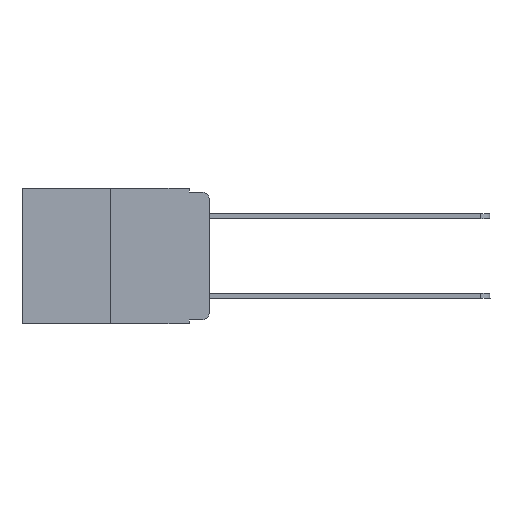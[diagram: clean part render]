
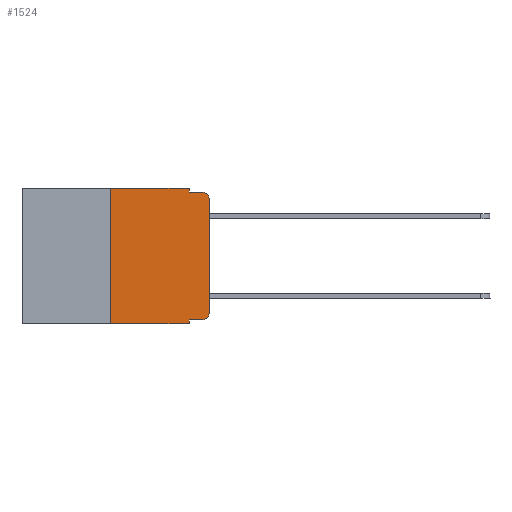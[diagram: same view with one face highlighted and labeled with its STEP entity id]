
A CAD part, left-side view. The second image highlights one B-rep face of the part: STEP entity #1524.
In plain terms, the highlighted planar face has unit normal (-1, 0, 0).
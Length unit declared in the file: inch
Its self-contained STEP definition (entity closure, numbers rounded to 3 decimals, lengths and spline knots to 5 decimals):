
#225 = CARTESIAN_POINT ( 'NONE',  ( 0., 0.473, -0.343 ) ) ;
#423 = VECTOR ( 'NONE', #4324, 39.37008 ) ;
#440 = VERTEX_POINT ( 'NONE', #7628 ) ;
#441 = VERTEX_POINT ( 'NONE', #1644 ) ;
#638 = DIRECTION ( 'NONE',  ( 0., -1., 0. ) ) ;
#814 = AXIS2_PLACEMENT_3D ( 'NONE', #3698, #3149, #5276 ) ;
#901 = EDGE_CURVE ( 'NONE', #3537, #441, #5194, .T. ) ;
#906 = AXIS2_PLACEMENT_3D ( 'NONE', #5093, #6842, #1493 ) ;
#969 = LINE ( 'NONE', #225, #7710 ) ;
#971 = CARTESIAN_POINT ( 'NONE',  ( 0., 0.051, -0.343 ) ) ;
#973 = CARTESIAN_POINT ( 'NONE',  ( 0., 0.051, 0. ) ) ;
#1084 = ORIENTED_EDGE ( 'NONE', *, *, #901, .F. ) ;
#1113 = VECTOR ( 'NONE', #3152, 39.37008 ) ;
#1220 = DIRECTION ( 'NONE',  ( 0., 0., 1. ) ) ;
#1253 = CARTESIAN_POINT ( 'NONE',  ( 0., 0.051, 0. ) ) ;
#1366 = CARTESIAN_POINT ( 'NONE',  ( 0., 0.25, 0. ) ) ;
#1490 = VECTOR ( 'NONE', #6040, 39.37008 ) ;
#1493 = DIRECTION ( 'NONE',  ( 0., 0., -1. ) ) ;
#1524 = ADVANCED_FACE ( 'NONE', ( #7562 ), #6873, .F. ) ;
#1567 = LINE ( 'NONE', #7398, #5049 ) ;
#1644 = CARTESIAN_POINT ( 'NONE',  ( 0., 0.02, -0.01 ) ) ;
#1646 = VERTEX_POINT ( 'NONE', #3939 ) ;
#1911 = VERTEX_POINT ( 'NONE', #9131 ) ;
#1951 = ORIENTED_EDGE ( 'NONE', *, *, #9587, .T. ) ;
#2141 = ORIENTED_EDGE ( 'NONE', *, *, #3349, .F. ) ;
#2215 = EDGE_CURVE ( 'NONE', #1646, #7354, #3371, .T. ) ;
#2324 = CIRCLE ( 'NONE', #5000, 0.02 ) ;
#2403 = LINE ( 'NONE', #5411, #6417 ) ;
#2621 = CIRCLE ( 'NONE', #906, 0.02 ) ;
#2812 = CARTESIAN_POINT ( 'NONE',  ( 0., 0., -0.03 ) ) ;
#2906 = EDGE_CURVE ( 'NONE', #440, #8587, #9098, .T. ) ;
#2920 = CARTESIAN_POINT ( 'NONE',  ( 0., 0.25, -0.343 ) ) ;
#3149 = DIRECTION ( 'NONE',  ( 1., 0., 0. ) ) ;
#3152 = DIRECTION ( 'NONE',  ( 0., -1., 0. ) ) ;
#3173 = DIRECTION ( 'NONE',  ( 0., -1., 0. ) ) ;
#3349 = EDGE_CURVE ( 'NONE', #8587, #3537, #2403, .T. ) ;
#3371 = LINE ( 'NONE', #1253, #3617 ) ;
#3537 = VERTEX_POINT ( 'NONE', #7972 ) ;
#3567 = DIRECTION ( 'NONE',  ( 0., 0., -1. ) ) ;
#3617 = VECTOR ( 'NONE', #3567, 39.37008 ) ;
#3698 = CARTESIAN_POINT ( 'NONE',  ( 0., 0.473, 0. ) ) ;
#3939 = CARTESIAN_POINT ( 'NONE',  ( 0., 0.051, -0.333 ) ) ;
#4218 = LINE ( 'NONE', #1366, #6331 ) ;
#4324 = DIRECTION ( 'NONE',  ( 0., 0., 1. ) ) ;
#4718 = ORIENTED_EDGE ( 'NONE', *, *, #6082, .T. ) ;
#4877 = ORIENTED_EDGE ( 'NONE', *, *, #8855, .T. ) ;
#5000 = AXIS2_PLACEMENT_3D ( 'NONE', #6572, #7211, #6618 ) ;
#5049 = VECTOR ( 'NONE', #638, 39.37008 ) ;
#5093 = CARTESIAN_POINT ( 'NONE',  ( 0., 0.02, -0.313 ) ) ;
#5194 = LINE ( 'NONE', #6683, #1490 ) ;
#5276 = DIRECTION ( 'NONE',  ( 0., 0., -1. ) ) ;
#5411 = CARTESIAN_POINT ( 'NONE',  ( 0., 0.051, 0. ) ) ;
#5592 = ORIENTED_EDGE ( 'NONE', *, *, #2215, .F. ) ;
#6040 = DIRECTION ( 'NONE',  ( 0., -1., 0. ) ) ;
#6082 = EDGE_CURVE ( 'NONE', #8847, #7354, #969, .T. ) ;
#6331 = VECTOR ( 'NONE', #1220, 39.37008 ) ;
#6417 = VECTOR ( 'NONE', #8440, 39.37008 ) ;
#6572 = CARTESIAN_POINT ( 'NONE',  ( 0., 0.02, -0.03 ) ) ;
#6618 = DIRECTION ( 'NONE',  ( 0., 0., -1. ) ) ;
#6625 = EDGE_CURVE ( 'NONE', #8847, #440, #4218, .T. ) ;
#6678 = CARTESIAN_POINT ( 'NONE',  ( 0., 0., 0. ) ) ;
#6683 = CARTESIAN_POINT ( 'NONE',  ( 0., 0.051, -0.01 ) ) ;
#6786 = EDGE_CURVE ( 'NONE', #1646, #7023, #1567, .T. ) ;
#6842 = DIRECTION ( 'NONE',  ( -1., 0., 0. ) ) ;
#6873 = PLANE ( 'NONE',  #814 ) ;
#6973 = CARTESIAN_POINT ( 'NONE',  ( 0., 0.473, 0. ) ) ;
#7023 = VERTEX_POINT ( 'NONE', #8727 ) ;
#7044 = ORIENTED_EDGE ( 'NONE', *, *, #6786, .T. ) ;
#7143 = ORIENTED_EDGE ( 'NONE', *, *, #6625, .F. ) ;
#7211 = DIRECTION ( 'NONE',  ( -1., 0., 0. ) ) ;
#7309 = LINE ( 'NONE', #6678, #423 ) ;
#7354 = VERTEX_POINT ( 'NONE', #971 ) ;
#7398 = CARTESIAN_POINT ( 'NONE',  ( 0., 0.051, -0.333 ) ) ;
#7562 = FACE_OUTER_BOUND ( 'NONE', #9254, .T. ) ;
#7628 = CARTESIAN_POINT ( 'NONE',  ( 0., 0.25, 0. ) ) ;
#7710 = VECTOR ( 'NONE', #3173, 39.37008 ) ;
#7972 = CARTESIAN_POINT ( 'NONE',  ( 0., 0.051, -0.01 ) ) ;
#7987 = VERTEX_POINT ( 'NONE', #2812 ) ;
#8065 = EDGE_CURVE ( 'NONE', #1911, #7987, #7309, .T. ) ;
#8440 = DIRECTION ( 'NONE',  ( 0., 0., -1. ) ) ;
#8587 = VERTEX_POINT ( 'NONE', #973 ) ;
#8727 = CARTESIAN_POINT ( 'NONE',  ( 0., 0.02, -0.333 ) ) ;
#8847 = VERTEX_POINT ( 'NONE', #2920 ) ;
#8855 = EDGE_CURVE ( 'NONE', #7023, #1911, #2621, .T. ) ;
#9098 = LINE ( 'NONE', #6973, #1113 ) ;
#9131 = CARTESIAN_POINT ( 'NONE',  ( 0., 0., -0.313 ) ) ;
#9254 = EDGE_LOOP ( 'NONE', ( #9288, #1951, #1084, #2141, #9489, #7143, #4718, #5592, #7044, #4877 ) ) ;
#9288 = ORIENTED_EDGE ( 'NONE', *, *, #8065, .T. ) ;
#9489 = ORIENTED_EDGE ( 'NONE', *, *, #2906, .F. ) ;
#9587 = EDGE_CURVE ( 'NONE', #7987, #441, #2324, .T. ) ;
